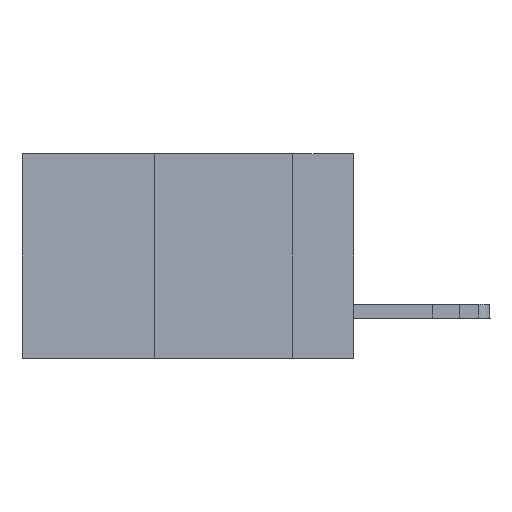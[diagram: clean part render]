
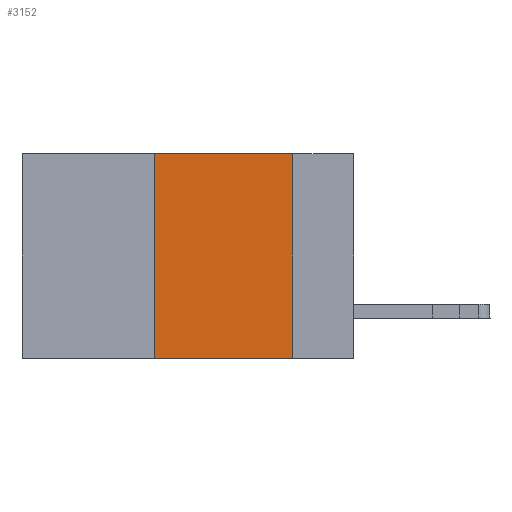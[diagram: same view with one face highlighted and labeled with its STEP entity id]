
A CAD part, left-side view. The second image highlights one B-rep face of the part: STEP entity #3152.
In plain terms, the highlighted planar face has unit normal (-1, 0, 0).
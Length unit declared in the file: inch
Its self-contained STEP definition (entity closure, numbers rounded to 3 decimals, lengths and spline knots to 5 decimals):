
#543 = DIRECTION ( 'NONE',  ( 0., 0., -1. ) ) ;
#761 = FACE_OUTER_BOUND ( 'NONE', #12624, .T. ) ;
#1946 = CARTESIAN_POINT ( 'NONE',  ( 0., 0.6, -0.37 ) ) ;
#2645 = VERTEX_POINT ( 'NONE', #9695 ) ;
#3152 = ADVANCED_FACE ( 'NONE', ( #761 ), #15499, .F. ) ;
#3192 = CARTESIAN_POINT ( 'NONE',  ( 0., 0.11, 0. ) ) ;
#3279 = CARTESIAN_POINT ( 'NONE',  ( 0., 0.36, -0.37 ) ) ;
#3294 = DIRECTION ( 'NONE',  ( 0., -1., 0. ) ) ;
#4009 = VECTOR ( 'NONE', #14906, 39.37008 ) ;
#4449 = VECTOR ( 'NONE', #11905, 39.37008 ) ;
#4685 = CARTESIAN_POINT ( 'NONE',  ( 0., 0.11, -0.37 ) ) ;
#4984 = VECTOR ( 'NONE', #3294, 39.37008 ) ;
#6314 = CARTESIAN_POINT ( 'NONE',  ( 0., 0.36, 0. ) ) ;
#6559 = VERTEX_POINT ( 'NONE', #8252 ) ;
#6836 = LINE ( 'NONE', #7610, #4009 ) ;
#6875 = ORIENTED_EDGE ( 'NONE', *, *, #13229, .F. ) ;
#6890 = ORIENTED_EDGE ( 'NONE', *, *, #15105, .T. ) ;
#7610 = CARTESIAN_POINT ( 'NONE',  ( 0., 0.6, 0. ) ) ;
#8214 = DIRECTION ( 'NONE',  ( 1., 0., 0. ) ) ;
#8252 = CARTESIAN_POINT ( 'NONE',  ( 0., 0.11, 0. ) ) ;
#8261 = ORIENTED_EDGE ( 'NONE', *, *, #11136, .F. ) ;
#8450 = ORIENTED_EDGE ( 'NONE', *, *, #14112, .F. ) ;
#9086 = LINE ( 'NONE', #1946, #4984 ) ;
#9695 = CARTESIAN_POINT ( 'NONE',  ( 0., 0.36, 0. ) ) ;
#9740 = VERTEX_POINT ( 'NONE', #4685 ) ;
#10011 = LINE ( 'NONE', #6314, #15678 ) ;
#10079 = DIRECTION ( 'NONE',  ( 0., 0., 1. ) ) ;
#11136 = EDGE_CURVE ( 'NONE', #13820, #2645, #10011, .T. ) ;
#11905 = DIRECTION ( 'NONE',  ( 0., 0., -1. ) ) ;
#12624 = EDGE_LOOP ( 'NONE', ( #6875, #8450, #8261, #6890 ) ) ;
#13229 = EDGE_CURVE ( 'NONE', #6559, #9740, #13554, .T. ) ;
#13296 = AXIS2_PLACEMENT_3D ( 'NONE', #15444, #8214, #543 ) ;
#13554 = LINE ( 'NONE', #3192, #4449 ) ;
#13820 = VERTEX_POINT ( 'NONE', #3279 ) ;
#14112 = EDGE_CURVE ( 'NONE', #2645, #6559, #6836, .T. ) ;
#14906 = DIRECTION ( 'NONE',  ( 0., -1., 0. ) ) ;
#15105 = EDGE_CURVE ( 'NONE', #13820, #9740, #9086, .T. ) ;
#15444 = CARTESIAN_POINT ( 'NONE',  ( 0., 0.6, 0. ) ) ;
#15499 = PLANE ( 'NONE',  #13296 ) ;
#15678 = VECTOR ( 'NONE', #10079, 39.37008 ) ;
